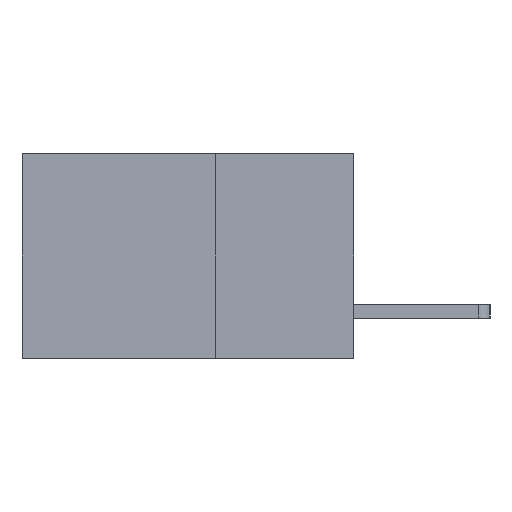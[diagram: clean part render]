
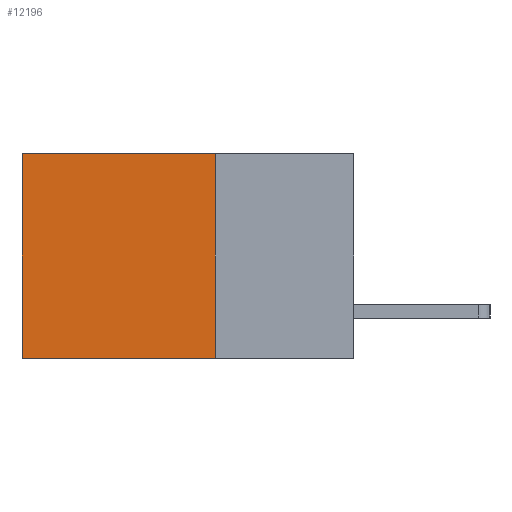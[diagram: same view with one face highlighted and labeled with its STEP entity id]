
A CAD part, left-side view. The second image highlights one B-rep face of the part: STEP entity #12196.
In plain terms, the highlighted planar face has unit normal (-1, 0, 0).
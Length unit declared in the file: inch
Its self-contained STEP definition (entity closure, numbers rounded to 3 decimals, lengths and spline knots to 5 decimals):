
#127 = ORIENTED_EDGE ( 'NONE', *, *, #2581, .F. ) ;
#387 = CARTESIAN_POINT ( 'NONE',  ( 0.2875, 0.6, 0. ) ) ;
#1165 = LINE ( 'NONE', #4193, #12246 ) ;
#2168 = AXIS2_PLACEMENT_3D ( 'NONE', #3294, #3434, #3365 ) ;
#2186 = VERTEX_POINT ( 'NONE', #9189 ) ;
#2581 = EDGE_CURVE ( 'NONE', #7725, #12240, #8681, .T. ) ;
#2651 = ORIENTED_EDGE ( 'NONE', *, *, #8509, .T. ) ;
#2774 = EDGE_LOOP ( 'NONE', ( #2651, #127, #8701, #7095 ) ) ;
#2994 = VECTOR ( 'NONE', #9847, 39.37008 ) ;
#3294 = CARTESIAN_POINT ( 'NONE',  ( 0.2875, 0.25, 0. ) ) ;
#3365 = DIRECTION ( 'NONE',  ( 0., 0., -1. ) ) ;
#3434 = DIRECTION ( 'NONE',  ( 1., 0., 0. ) ) ;
#4111 = VERTEX_POINT ( 'NONE', #8406 ) ;
#4193 = CARTESIAN_POINT ( 'NONE',  ( 0.2875, 0.25, 0. ) ) ;
#4278 = CARTESIAN_POINT ( 'NONE',  ( 0.2875, 0.6, -0.37 ) ) ;
#4713 = EDGE_CURVE ( 'NONE', #4111, #7725, #5025, .T. ) ;
#5008 = VECTOR ( 'NONE', #9486, 39.37008 ) ;
#5025 = LINE ( 'NONE', #10882, #2994 ) ;
#5211 = EDGE_CURVE ( 'NONE', #4111, #2186, #1165, .T. ) ;
#6675 = CARTESIAN_POINT ( 'NONE',  ( 0.2875, 0.25, -0.37 ) ) ;
#7095 = ORIENTED_EDGE ( 'NONE', *, *, #5211, .T. ) ;
#7525 = LINE ( 'NONE', #387, #5008 ) ;
#7725 = VERTEX_POINT ( 'NONE', #10189 ) ;
#7803 = VECTOR ( 'NONE', #12663, 39.37008 ) ;
#8243 = DIRECTION ( 'NONE',  ( 0., 1., 0. ) ) ;
#8406 = CARTESIAN_POINT ( 'NONE',  ( 0.2875, 0.25, 0. ) ) ;
#8509 = EDGE_CURVE ( 'NONE', #2186, #12240, #7525, .T. ) ;
#8681 = LINE ( 'NONE', #6675, #7803 ) ;
#8701 = ORIENTED_EDGE ( 'NONE', *, *, #4713, .F. ) ;
#8999 = PLANE ( 'NONE',  #2168 ) ;
#9189 = CARTESIAN_POINT ( 'NONE',  ( 0.2875, 0.6, 0. ) ) ;
#9486 = DIRECTION ( 'NONE',  ( 0., 0., -1. ) ) ;
#9847 = DIRECTION ( 'NONE',  ( 0., 0., -1. ) ) ;
#10189 = CARTESIAN_POINT ( 'NONE',  ( 0.2875, 0.25, -0.37 ) ) ;
#10882 = CARTESIAN_POINT ( 'NONE',  ( 0.2875, 0.25, 0. ) ) ;
#10933 = FACE_OUTER_BOUND ( 'NONE', #2774, .T. ) ;
#12196 = ADVANCED_FACE ( 'NONE', ( #10933 ), #8999, .F. ) ;
#12240 = VERTEX_POINT ( 'NONE', #4278 ) ;
#12246 = VECTOR ( 'NONE', #8243, 39.37008 ) ;
#12663 = DIRECTION ( 'NONE',  ( 0., 1., 0. ) ) ;
